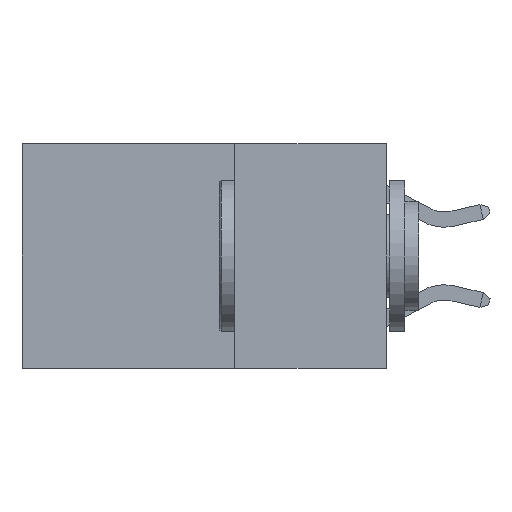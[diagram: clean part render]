
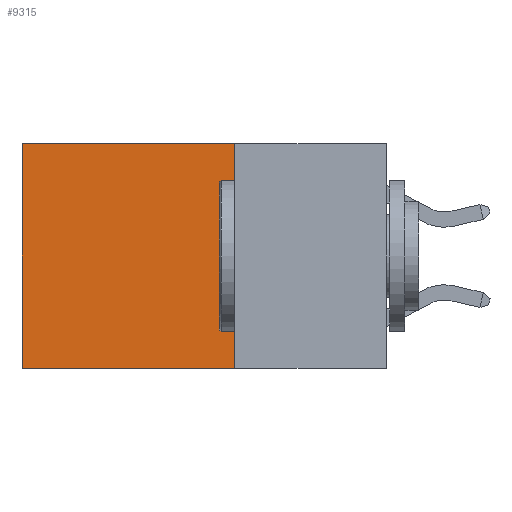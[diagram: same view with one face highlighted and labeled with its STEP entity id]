
A CAD part, left-side view. The second image highlights one B-rep face of the part: STEP entity #9315.
In plain terms, the highlighted planar face has unit normal (-1, 0, 0).
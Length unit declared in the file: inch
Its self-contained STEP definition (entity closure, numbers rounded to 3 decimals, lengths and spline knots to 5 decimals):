
#25 = VERTEX_POINT ( 'NONE', #22329 ) ;
#203 = CARTESIAN_POINT ( 'NONE',  ( 0.2625, 0.25, 0. ) ) ;
#800 = VERTEX_POINT ( 'NONE', #26045 ) ;
#2184 = DIRECTION ( 'NONE',  ( 0., 1., 0. ) ) ;
#2871 = ORIENTED_EDGE ( 'NONE', *, *, #17562, .F. ) ;
#2949 = DIRECTION ( 'NONE',  ( 0., 0., -1. ) ) ;
#3629 = EDGE_CURVE ( 'NONE', #25, #23780, #12336, .T. ) ;
#4280 = EDGE_CURVE ( 'NONE', #25, #13088, #16727, .T. ) ;
#4868 = CARTESIAN_POINT ( 'NONE',  ( 0.2625, 0.6, 0. ) ) ;
#6854 = DIRECTION ( 'NONE',  ( 0., 0., -1. ) ) ;
#7606 = ORIENTED_EDGE ( 'NONE', *, *, #4280, .T. ) ;
#8802 = EDGE_LOOP ( 'NONE', ( #25574, #2871, #23422, #7606 ) ) ;
#8998 = CARTESIAN_POINT ( 'NONE',  ( 0.2625, 0.25, -0.37 ) ) ;
#9315 = ADVANCED_FACE ( 'NONE', ( #21457 ), #10422, .F. ) ;
#10422 = PLANE ( 'NONE',  #22856 ) ;
#12336 = LINE ( 'NONE', #24802, #20254 ) ;
#13088 = VERTEX_POINT ( 'NONE', #4868 ) ;
#13443 = DIRECTION ( 'NONE',  ( 0., 1., 0. ) ) ;
#15787 = CARTESIAN_POINT ( 'NONE',  ( 0.2625, 0.6, 0. ) ) ;
#16209 = EDGE_CURVE ( 'NONE', #13088, #800, #25510, .T. ) ;
#16727 = LINE ( 'NONE', #203, #23074 ) ;
#17562 = EDGE_CURVE ( 'NONE', #23780, #800, #21161, .T. ) ;
#18623 = DIRECTION ( 'NONE',  ( 0., 0., -1. ) ) ;
#18924 = DIRECTION ( 'NONE',  ( 1., 0., 0. ) ) ;
#20254 = VECTOR ( 'NONE', #18623, 39.37008 ) ;
#21161 = LINE ( 'NONE', #8998, #23893 ) ;
#21457 = FACE_OUTER_BOUND ( 'NONE', #8802, .T. ) ;
#22329 = CARTESIAN_POINT ( 'NONE',  ( 0.2625, 0.25, 0. ) ) ;
#22522 = VECTOR ( 'NONE', #2949, 39.37008 ) ;
#22690 = CARTESIAN_POINT ( 'NONE',  ( 0.2625, 0.25, -0.37 ) ) ;
#22856 = AXIS2_PLACEMENT_3D ( 'NONE', #23246, #18924, #6854 ) ;
#23074 = VECTOR ( 'NONE', #2184, 39.37008 ) ;
#23246 = CARTESIAN_POINT ( 'NONE',  ( 0.2625, 0.25, 0. ) ) ;
#23422 = ORIENTED_EDGE ( 'NONE', *, *, #3629, .F. ) ;
#23780 = VERTEX_POINT ( 'NONE', #22690 ) ;
#23893 = VECTOR ( 'NONE', #13443, 39.37008 ) ;
#24802 = CARTESIAN_POINT ( 'NONE',  ( 0.2625, 0.25, 0. ) ) ;
#25510 = LINE ( 'NONE', #15787, #22522 ) ;
#25574 = ORIENTED_EDGE ( 'NONE', *, *, #16209, .T. ) ;
#26045 = CARTESIAN_POINT ( 'NONE',  ( 0.2625, 0.6, -0.37 ) ) ;
